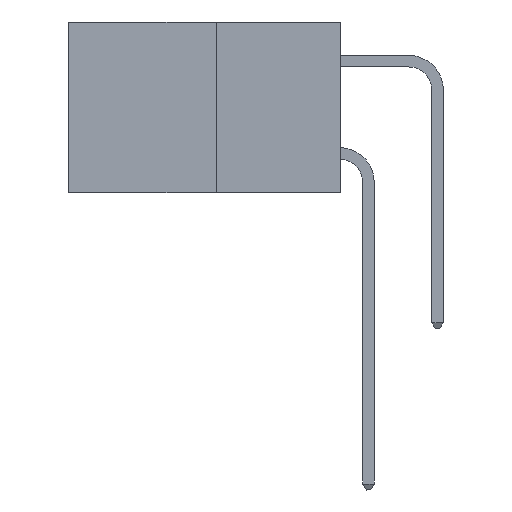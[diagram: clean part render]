
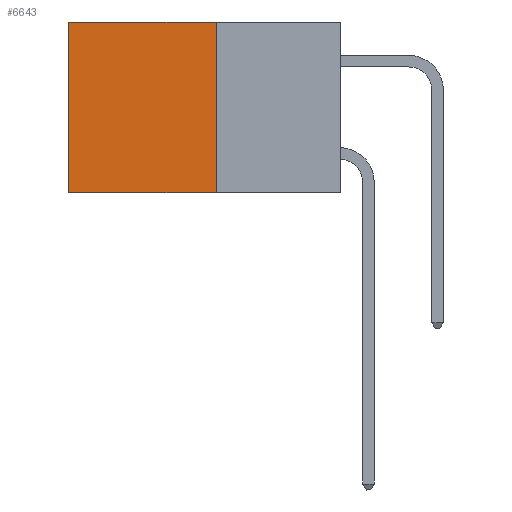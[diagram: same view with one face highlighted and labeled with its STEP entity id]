
A CAD part, left-side view. The second image highlights one B-rep face of the part: STEP entity #6643.
In plain terms, the highlighted planar face has unit normal (-1, 0, 0).
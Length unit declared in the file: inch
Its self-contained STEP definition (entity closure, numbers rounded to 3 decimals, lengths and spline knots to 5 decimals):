
#189 = LINE ( 'NONE', #7501, #5445 ) ;
#593 = EDGE_CURVE ( 'NONE', #5850, #4972, #189, .T. ) ;
#750 = CARTESIAN_POINT ( 'NONE',  ( 0.277, 0.27, -0.37 ) ) ;
#1039 = FACE_OUTER_BOUND ( 'NONE', #2035, .T. ) ;
#1614 = VECTOR ( 'NONE', #3689, 39.37008 ) ;
#1824 = CARTESIAN_POINT ( 'NONE',  ( 0.277, 0.59, -0.37 ) ) ;
#1988 = LINE ( 'NONE', #9227, #5587 ) ;
#2035 = EDGE_LOOP ( 'NONE', ( #8876, #10519, #5709, #3618 ) ) ;
#2633 = EDGE_CURVE ( 'NONE', #4972, #9677, #1988, .T. ) ;
#2752 = CARTESIAN_POINT ( 'NONE',  ( 0.277, 0.27, -0.37 ) ) ;
#3543 = CARTESIAN_POINT ( 'NONE',  ( 0.277, 0.59, 0. ) ) ;
#3612 = DIRECTION ( 'NONE',  ( 0., 0., -1. ) ) ;
#3618 = ORIENTED_EDGE ( 'NONE', *, *, #593, .T. ) ;
#3667 = VECTOR ( 'NONE', #9611, 39.37008 ) ;
#3689 = DIRECTION ( 'NONE',  ( 0., 1., 0. ) ) ;
#3846 = PLANE ( 'NONE',  #8856 ) ;
#4972 = VERTEX_POINT ( 'NONE', #3543 ) ;
#5057 = CARTESIAN_POINT ( 'NONE',  ( 0.277, 0.27, -0.37 ) ) ;
#5136 = VERTEX_POINT ( 'NONE', #750 ) ;
#5445 = VECTOR ( 'NONE', #8139, 39.37008 ) ;
#5587 = VECTOR ( 'NONE', #3612, 39.37008 ) ;
#5608 = DIRECTION ( 'NONE',  ( 1., 0., 0. ) ) ;
#5709 = ORIENTED_EDGE ( 'NONE', *, *, #9282, .F. ) ;
#5816 = EDGE_CURVE ( 'NONE', #5136, #9677, #6268, .T. ) ;
#5850 = VERTEX_POINT ( 'NONE', #11042 ) ;
#6268 = LINE ( 'NONE', #2752, #1614 ) ;
#6643 = ADVANCED_FACE ( 'NONE', ( #1039 ), #3846, .F. ) ;
#7501 = CARTESIAN_POINT ( 'NONE',  ( 0.277, 0.27, 0. ) ) ;
#8139 = DIRECTION ( 'NONE',  ( 0., 1., 0. ) ) ;
#8856 = AXIS2_PLACEMENT_3D ( 'NONE', #11138, #5608, #11979 ) ;
#8876 = ORIENTED_EDGE ( 'NONE', *, *, #2633, .T. ) ;
#9227 = CARTESIAN_POINT ( 'NONE',  ( 0.277, 0.59, -0.37 ) ) ;
#9282 = EDGE_CURVE ( 'NONE', #5850, #5136, #11237, .T. ) ;
#9611 = DIRECTION ( 'NONE',  ( 0., 0., -1. ) ) ;
#9677 = VERTEX_POINT ( 'NONE', #1824 ) ;
#10519 = ORIENTED_EDGE ( 'NONE', *, *, #5816, .F. ) ;
#11042 = CARTESIAN_POINT ( 'NONE',  ( 0.277, 0.27, 0. ) ) ;
#11138 = CARTESIAN_POINT ( 'NONE',  ( 0.277, 0.27, -0.37 ) ) ;
#11237 = LINE ( 'NONE', #5057, #3667 ) ;
#11979 = DIRECTION ( 'NONE',  ( 0., 0., -1. ) ) ;
